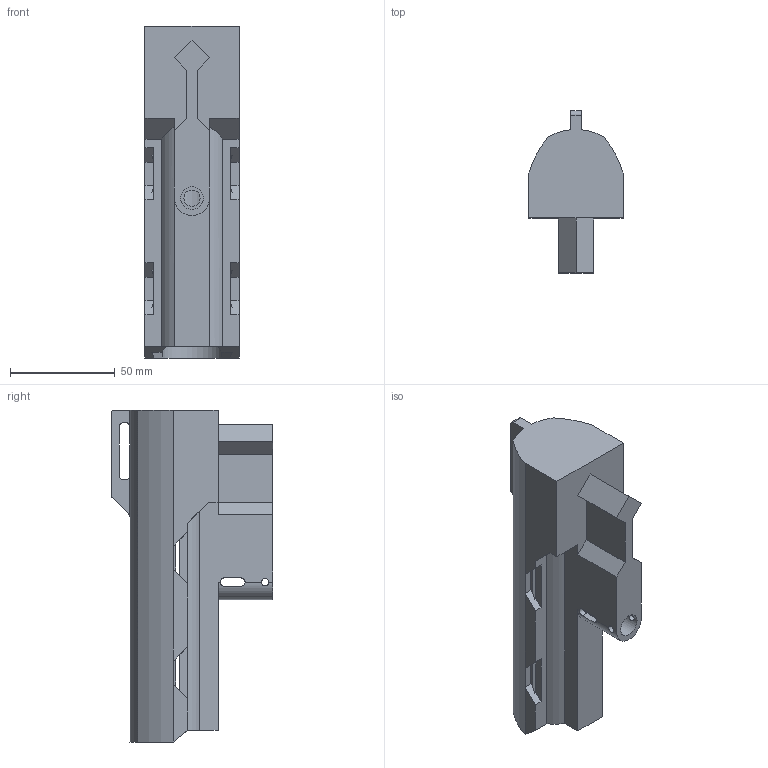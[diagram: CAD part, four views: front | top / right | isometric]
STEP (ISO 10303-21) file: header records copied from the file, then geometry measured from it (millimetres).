
FILE_DESCRIPTION( ( '' ), ' ' );
FILE_NAME( '5dc6e2d694333712756285f8.step', '2019-11-09T16:01:26', ( '' ), ( '' ), ' ', ' ', ' ' );
FILE_SCHEMA( ( 'AUTOMOTIVE_DESIGN { 1 0 10303 214 1 1 1 1 }' ) );
Length unit declared in the file: metre
Products named in the file (1): Part 1
Bounding box: 45 x 77.46 x 158.75 mm (x, y, z)
Volume: 106559.2 mm3; surface area: 52607 mm2
Topology: 1 solids, 1 shells, 97 faces, 309 edges, 201 vertices
Faces by surface type: plane 72, cylinder 22, cone 1, bspline 1, torus 1
Full cylindrical faces by diameter (mm): 3.5 x2, 7.75 x1, 11 x1
Entity records: 4528 total; most frequent: CARTESIAN_POINT 1019, ORIENTED_EDGE 604, DIRECTION 519, EDGE_CURVE 302, LINE 239, VECTOR 239, VERTEX_POINT 198, AXIS2_PLACEMENT_3D 140
